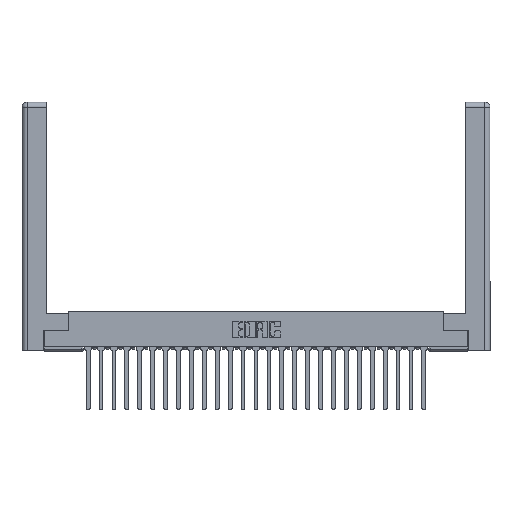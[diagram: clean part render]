
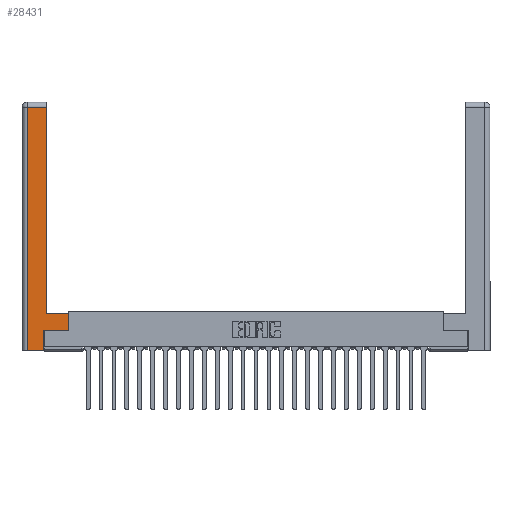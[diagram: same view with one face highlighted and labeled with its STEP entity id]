
A CAD part, top view. The second image highlights one B-rep face of the part: STEP entity #28431.
In plain terms, the highlighted planar face has unit normal (0, 0, 1).
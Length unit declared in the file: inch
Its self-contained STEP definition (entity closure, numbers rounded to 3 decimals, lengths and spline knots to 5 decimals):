
#386 = VERTEX_POINT ( 'NONE', #3462 ) ;
#2147 = DIRECTION ( 'NONE',  ( 0., -1., 0. ) ) ;
#2455 = VECTOR ( 'NONE', #17996, 39.37008 ) ;
#2598 = VERTEX_POINT ( 'NONE', #27179 ) ;
#2716 = CARTESIAN_POINT ( 'NONE',  ( 0.0615, 2.94, 0. ) ) ;
#2846 = CARTESIAN_POINT ( 'NONE',  ( 0.265, 0., 0. ) ) ;
#3020 = LINE ( 'NONE', #24594, #26024 ) ;
#3183 = DIRECTION ( 'NONE',  ( 0., 1., 0. ) ) ;
#3368 = CARTESIAN_POINT ( 'NONE',  ( 0.265, 0.245, 0. ) ) ;
#3462 = CARTESIAN_POINT ( 'NONE',  ( 0.295, 2.94, 0. ) ) ;
#4174 = LINE ( 'NONE', #20513, #18304 ) ;
#4539 = CARTESIAN_POINT ( 'NONE',  ( 0.0615, 0., 0. ) ) ;
#4730 = CARTESIAN_POINT ( 'NONE',  ( 0.295, 0.45, 0. ) ) ;
#5090 = LINE ( 'NONE', #5156, #11584 ) ;
#5156 = CARTESIAN_POINT ( 'NONE',  ( 0.565, 0.45, 0. ) ) ;
#5238 = CARTESIAN_POINT ( 'NONE',  ( 0.565, 0.245, 0. ) ) ;
#6229 = LINE ( 'NONE', #4730, #2455 ) ;
#6270 = EDGE_CURVE ( 'NONE', #386, #12774, #4174, .T. ) ;
#6400 = DIRECTION ( 'NONE',  ( 1., 0., 0. ) ) ;
#6409 = LINE ( 'NONE', #21651, #17735 ) ;
#7737 = CARTESIAN_POINT ( 'NONE',  ( 0.295, 0.45, 0. ) ) ;
#8170 = CARTESIAN_POINT ( 'NONE',  ( 0., 0., 0. ) ) ;
#9587 = DIRECTION ( 'NONE',  ( 0., 1., 0. ) ) ;
#10719 = EDGE_LOOP ( 'NONE', ( #19581, #11825, #20422, #20884, #16436, #14080, #17945, #21766 ) ) ;
#11584 = VECTOR ( 'NONE', #9587, 39.37008 ) ;
#11630 = AXIS2_PLACEMENT_3D ( 'NONE', #8170, #19764, #21682 ) ;
#11716 = FACE_OUTER_BOUND ( 'NONE', #10719, .T. ) ;
#11825 = ORIENTED_EDGE ( 'NONE', *, *, #6270, .T. ) ;
#12192 = EDGE_CURVE ( 'NONE', #25242, #17647, #19908, .T. ) ;
#12216 = VERTEX_POINT ( 'NONE', #5238 ) ;
#12766 = LINE ( 'NONE', #4539, #18663 ) ;
#12774 = VERTEX_POINT ( 'NONE', #2716 ) ;
#13154 = VERTEX_POINT ( 'NONE', #19389 ) ;
#13442 = EDGE_CURVE ( 'NONE', #25682, #386, #3020, .T. ) ;
#13872 = EDGE_CURVE ( 'NONE', #2598, #12216, #6409, .T. ) ;
#14078 = VECTOR ( 'NONE', #27069, 39.37008 ) ;
#14080 = ORIENTED_EDGE ( 'NONE', *, *, #13872, .T. ) ;
#15162 = VECTOR ( 'NONE', #3183, 39.37008 ) ;
#15575 = EDGE_CURVE ( 'NONE', #12774, #25242, #12766, .T. ) ;
#15926 = EDGE_CURVE ( 'NONE', #17647, #2598, #26186, .T. ) ;
#16436 = ORIENTED_EDGE ( 'NONE', *, *, #15926, .T. ) ;
#17647 = VERTEX_POINT ( 'NONE', #20873 ) ;
#17735 = VECTOR ( 'NONE', #6400, 39.37008 ) ;
#17945 = ORIENTED_EDGE ( 'NONE', *, *, #19056, .T. ) ;
#17996 = DIRECTION ( 'NONE',  ( -1., 0., 0. ) ) ;
#18304 = VECTOR ( 'NONE', #24753, 39.37008 ) ;
#18444 = DIRECTION ( 'NONE',  ( 0., 1., 0. ) ) ;
#18663 = VECTOR ( 'NONE', #2147, 39.37008 ) ;
#19056 = EDGE_CURVE ( 'NONE', #12216, #13154, #5090, .T. ) ;
#19389 = CARTESIAN_POINT ( 'NONE',  ( 0.565, 0.45, 0. ) ) ;
#19581 = ORIENTED_EDGE ( 'NONE', *, *, #13442, .T. ) ;
#19764 = DIRECTION ( 'NONE',  ( 0., 0., -1. ) ) ;
#19908 = LINE ( 'NONE', #2846, #14078 ) ;
#20422 = ORIENTED_EDGE ( 'NONE', *, *, #15575, .T. ) ;
#20513 = CARTESIAN_POINT ( 'NONE',  ( 0.0615, 2.94, 0. ) ) ;
#20821 = CARTESIAN_POINT ( 'NONE',  ( 0.0615, 0., 0. ) ) ;
#20873 = CARTESIAN_POINT ( 'NONE',  ( 0.265, 0., 0. ) ) ;
#20884 = ORIENTED_EDGE ( 'NONE', *, *, #12192, .T. ) ;
#21651 = CARTESIAN_POINT ( 'NONE',  ( 0.565, 0.245, 0. ) ) ;
#21682 = DIRECTION ( 'NONE',  ( -1., 0., 0. ) ) ;
#21766 = ORIENTED_EDGE ( 'NONE', *, *, #27953, .T. ) ;
#23831 = PLANE ( 'NONE',  #11630 ) ;
#24594 = CARTESIAN_POINT ( 'NONE',  ( 0.295, 3., 0. ) ) ;
#24753 = DIRECTION ( 'NONE',  ( -1., 0., 0. ) ) ;
#25242 = VERTEX_POINT ( 'NONE', #20821 ) ;
#25682 = VERTEX_POINT ( 'NONE', #7737 ) ;
#26024 = VECTOR ( 'NONE', #18444, 39.37008 ) ;
#26186 = LINE ( 'NONE', #3368, #15162 ) ;
#27069 = DIRECTION ( 'NONE',  ( 1., 0., 0. ) ) ;
#27179 = CARTESIAN_POINT ( 'NONE',  ( 0.265, 0.245, 0. ) ) ;
#27953 = EDGE_CURVE ( 'NONE', #13154, #25682, #6229, .T. ) ;
#28431 = ADVANCED_FACE ( 'NONE', ( #11716 ), #23831, .F. ) ;
